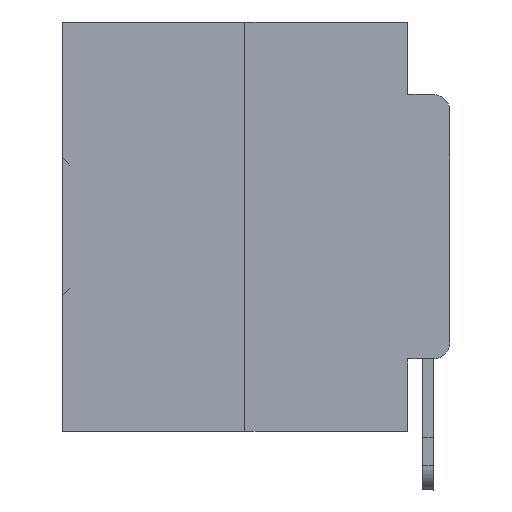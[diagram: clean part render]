
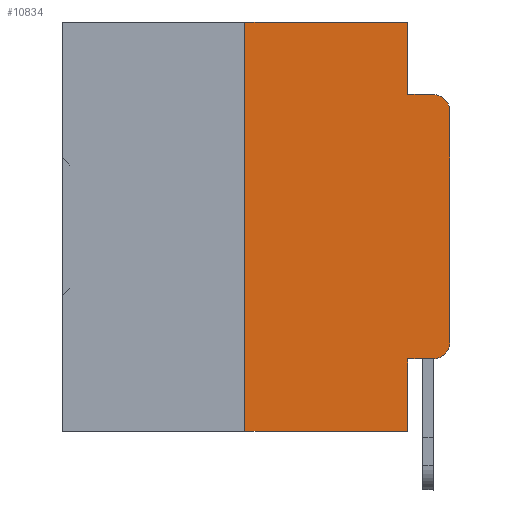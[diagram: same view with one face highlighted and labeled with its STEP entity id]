
A CAD part, left-side view. The second image highlights one B-rep face of the part: STEP entity #10834.
In plain terms, the highlighted planar face has unit normal (-1, 0, 0).
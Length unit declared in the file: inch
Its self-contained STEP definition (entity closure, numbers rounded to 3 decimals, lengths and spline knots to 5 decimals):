
#312 = ORIENTED_EDGE ( 'NONE', *, *, #14361, .F. ) ;
#470 = ORIENTED_EDGE ( 'NONE', *, *, #15045, .T. ) ;
#596 = DIRECTION ( 'NONE',  ( -1., 0., 0. ) ) ;
#1749 = ORIENTED_EDGE ( 'NONE', *, *, #10726, .F. ) ;
#2607 = ORIENTED_EDGE ( 'NONE', *, *, #34298, .T. ) ;
#2750 = VECTOR ( 'NONE', #7273, 39.37008 ) ;
#3465 = DIRECTION ( 'NONE',  ( 0., 0., -1. ) ) ;
#3646 = ORIENTED_EDGE ( 'NONE', *, *, #6159, .T. ) ;
#4305 = EDGE_LOOP ( 'NONE', ( #3646, #470, #312, #1749, #29534, #25371, #2607, #17227, #29997, #32813 ) ) ;
#4609 = EDGE_CURVE ( 'NONE', #35078, #11509, #15966, .T. ) ;
#4656 = CARTESIAN_POINT ( 'NONE',  ( 0., 0.02, -0.0885 ) ) ;
#5046 = CARTESIAN_POINT ( 'NONE',  ( 0., 0.051, -0.4115 ) ) ;
#5612 = EDGE_CURVE ( 'NONE', #5674, #35032, #25501, .T. ) ;
#5674 = VERTEX_POINT ( 'NONE', #31956 ) ;
#5888 = CARTESIAN_POINT ( 'NONE',  ( 0., 0., 0. ) ) ;
#6159 = EDGE_CURVE ( 'NONE', #35678, #27506, #26816, .T. ) ;
#6468 = CARTESIAN_POINT ( 'NONE',  ( 0., 0.473, 0. ) ) ;
#7273 = DIRECTION ( 'NONE',  ( 0., -1., 0. ) ) ;
#7356 = CARTESIAN_POINT ( 'NONE',  ( 0., 0.25, 0. ) ) ;
#8019 = DIRECTION ( 'NONE',  ( 1., 0., 0. ) ) ;
#10233 = FACE_OUTER_BOUND ( 'NONE', #4305, .T. ) ;
#10575 = LINE ( 'NONE', #24002, #2750 ) ;
#10726 = EDGE_CURVE ( 'NONE', #11509, #30763, #20747, .T. ) ;
#10773 = DIRECTION ( 'NONE',  ( 0., 0., 1. ) ) ;
#10792 = DIRECTION ( 'NONE',  ( 0., 0., -1. ) ) ;
#10834 = ADVANCED_FACE ( 'NONE', ( #10233 ), #16346, .F. ) ;
#10899 = VECTOR ( 'NONE', #10773, 39.37008 ) ;
#11285 = LINE ( 'NONE', #24623, #10899 ) ;
#11509 = VERTEX_POINT ( 'NONE', #30479 ) ;
#11977 = LINE ( 'NONE', #5046, #23849 ) ;
#12182 = CARTESIAN_POINT ( 'NONE',  ( 0., 0.051, -0.5 ) ) ;
#12357 = DIRECTION ( 'NONE',  ( 0., 0., -1. ) ) ;
#12421 = VERTEX_POINT ( 'NONE', #29832 ) ;
#12807 = VERTEX_POINT ( 'NONE', #4656 ) ;
#13910 = CARTESIAN_POINT ( 'NONE',  ( 0., 0., -0.1085 ) ) ;
#14361 = EDGE_CURVE ( 'NONE', #30763, #12807, #10575, .T. ) ;
#15045 = EDGE_CURVE ( 'NONE', #27506, #12807, #15800, .T. ) ;
#15800 = CIRCLE ( 'NONE', #21615, 0.02 ) ;
#15966 = LINE ( 'NONE', #6468, #28588 ) ;
#16114 = EDGE_CURVE ( 'NONE', #16176, #35078, #11285, .T. ) ;
#16176 = VERTEX_POINT ( 'NONE', #34703 ) ;
#16305 = DIRECTION ( 'NONE',  ( 0., -1., 0. ) ) ;
#16346 = PLANE ( 'NONE',  #34541 ) ;
#16889 = CARTESIAN_POINT ( 'NONE',  ( 0., 0.051, -0.0885 ) ) ;
#17193 = CIRCLE ( 'NONE', #21030, 0.02 ) ;
#17227 = ORIENTED_EDGE ( 'NONE', *, *, #5612, .F. ) ;
#18449 = EDGE_CURVE ( 'NONE', #5674, #12421, #11977, .T. ) ;
#19045 = VECTOR ( 'NONE', #31147, 39.37008 ) ;
#19382 = CARTESIAN_POINT ( 'NONE',  ( 0., 0.051, 0. ) ) ;
#19397 = EDGE_CURVE ( 'NONE', #12421, #35678, #17193, .T. ) ;
#20747 = LINE ( 'NONE', #24685, #19045 ) ;
#21030 = AXIS2_PLACEMENT_3D ( 'NONE', #34071, #596, #3465 ) ;
#21615 = AXIS2_PLACEMENT_3D ( 'NONE', #26324, #30145, #12357 ) ;
#23132 = DIRECTION ( 'NONE',  ( 0., -1., 0. ) ) ;
#23655 = CARTESIAN_POINT ( 'NONE',  ( 0., 0., -0.3915 ) ) ;
#23849 = VECTOR ( 'NONE', #16305, 39.37008 ) ;
#24002 = CARTESIAN_POINT ( 'NONE',  ( 0., 0.051, -0.0885 ) ) ;
#24623 = CARTESIAN_POINT ( 'NONE',  ( 0., 0.25, 0. ) ) ;
#24685 = CARTESIAN_POINT ( 'NONE',  ( 0., 0.051, 0. ) ) ;
#25371 = ORIENTED_EDGE ( 'NONE', *, *, #16114, .F. ) ;
#25501 = LINE ( 'NONE', #19382, #30709 ) ;
#25507 = LINE ( 'NONE', #28623, #36019 ) ;
#26243 = DIRECTION ( 'NONE',  ( 0., -1., 0. ) ) ;
#26324 = CARTESIAN_POINT ( 'NONE',  ( 0., 0.02, -0.1085 ) ) ;
#26816 = LINE ( 'NONE', #5888, #28115 ) ;
#27506 = VERTEX_POINT ( 'NONE', #13910 ) ;
#28115 = VECTOR ( 'NONE', #28125, 39.37008 ) ;
#28125 = DIRECTION ( 'NONE',  ( 0., 0., 1. ) ) ;
#28588 = VECTOR ( 'NONE', #26243, 39.37008 ) ;
#28623 = CARTESIAN_POINT ( 'NONE',  ( 0., 0.473, -0.5 ) ) ;
#29534 = ORIENTED_EDGE ( 'NONE', *, *, #4609, .F. ) ;
#29832 = CARTESIAN_POINT ( 'NONE',  ( 0., 0.02, -0.4115 ) ) ;
#29997 = ORIENTED_EDGE ( 'NONE', *, *, #18449, .T. ) ;
#30145 = DIRECTION ( 'NONE',  ( -1., 0., 0. ) ) ;
#30479 = CARTESIAN_POINT ( 'NONE',  ( 0., 0.051, 0. ) ) ;
#30709 = VECTOR ( 'NONE', #34121, 39.37008 ) ;
#30763 = VERTEX_POINT ( 'NONE', #16889 ) ;
#31147 = DIRECTION ( 'NONE',  ( 0., 0., -1. ) ) ;
#31956 = CARTESIAN_POINT ( 'NONE',  ( 0., 0.051, -0.4115 ) ) ;
#32813 = ORIENTED_EDGE ( 'NONE', *, *, #19397, .T. ) ;
#34071 = CARTESIAN_POINT ( 'NONE',  ( 0., 0.02, -0.3915 ) ) ;
#34121 = DIRECTION ( 'NONE',  ( 0., 0., -1. ) ) ;
#34298 = EDGE_CURVE ( 'NONE', #16176, #35032, #25507, .T. ) ;
#34541 = AXIS2_PLACEMENT_3D ( 'NONE', #35840, #8019, #10792 ) ;
#34703 = CARTESIAN_POINT ( 'NONE',  ( 0., 0.25, -0.5 ) ) ;
#35032 = VERTEX_POINT ( 'NONE', #12182 ) ;
#35078 = VERTEX_POINT ( 'NONE', #7356 ) ;
#35678 = VERTEX_POINT ( 'NONE', #23655 ) ;
#35840 = CARTESIAN_POINT ( 'NONE',  ( 0., 0.473, 0. ) ) ;
#36019 = VECTOR ( 'NONE', #23132, 39.37008 ) ;
